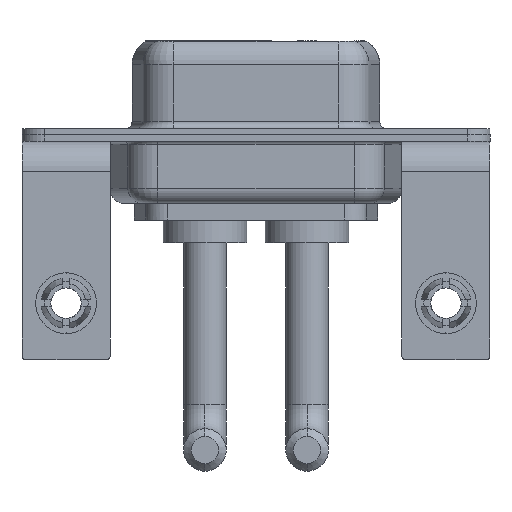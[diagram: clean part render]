
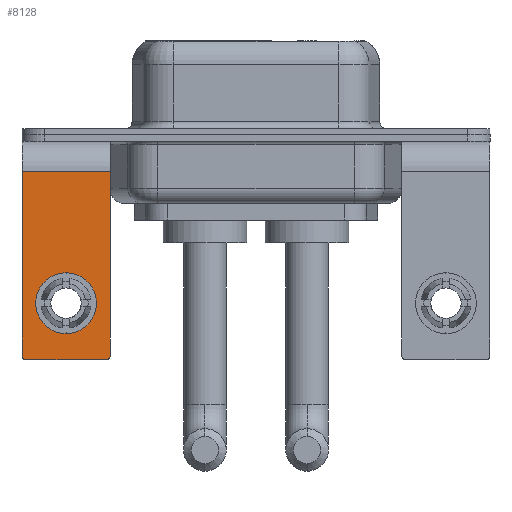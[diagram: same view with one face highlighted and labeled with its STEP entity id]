
A CAD part, front view. The second image highlights one B-rep face of the part: STEP entity #8128.
In plain terms, the highlighted planar face has unit normal (0, -1, 0).
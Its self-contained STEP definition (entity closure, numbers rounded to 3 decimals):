
#60 = VERTEX_POINT ( 'NONE', #4407 ) ;
#102 = EDGE_CURVE ( 'NONE', #496, #12610, #9292, .T. ) ;
#114 = ORIENTED_EDGE ( 'NONE', *, *, #12944, .T. ) ;
#496 = VERTEX_POINT ( 'NONE', #11418 ) ;
#649 = CIRCLE ( 'NONE', #12820, 2. ) ;
#994 = VERTEX_POINT ( 'NONE', #14543 ) ;
#1002 = DIRECTION ( 'NONE',  ( 0., 1., 0. ) ) ;
#1233 = ORIENTED_EDGE ( 'NONE', *, *, #102, .F. ) ;
#1258 = VERTEX_POINT ( 'NONE', #14523 ) ;
#1365 = DIRECTION ( 'NONE',  ( 0., 0., 1. ) ) ;
#1429 = EDGE_LOOP ( 'NONE', ( #15590, #114 ) ) ;
#1766 = ORIENTED_EDGE ( 'NONE', *, *, #7367, .T. ) ;
#1921 = CARTESIAN_POINT ( 'NONE',  ( 0., -6.25, -13.07 ) ) ;
#2092 = DIRECTION ( 'NONE',  ( -1., 0., 0. ) ) ;
#2646 = VECTOR ( 'NONE', #15547, 1000. ) ;
#2966 = CIRCLE ( 'NONE', #8007, 0.25 ) ;
#3191 = CIRCLE ( 'NONE', #12035, 0.25 ) ;
#3554 = EDGE_CURVE ( 'NONE', #1258, #60, #14537, .T. ) ;
#3587 = DIRECTION ( 'NONE',  ( 0., 0., -1. ) ) ;
#3794 = DIRECTION ( 'NONE',  ( 0., 0., 1. ) ) ;
#4407 = CARTESIAN_POINT ( 'NONE',  ( -2.9, -6.25, -2.4 ) ) ;
#4974 = CARTESIAN_POINT ( 'NONE',  ( 2.65, -6.25, -14.55 ) ) ;
#5122 = DIRECTION ( 'NONE',  ( 0., -1., 0. ) ) ;
#5253 = VECTOR ( 'NONE', #3587, 1000. ) ;
#6022 = EDGE_CURVE ( 'NONE', #496, #6179, #2966, .T. ) ;
#6058 = DIRECTION ( 'NONE',  ( 0., 0., 1. ) ) ;
#6179 = VERTEX_POINT ( 'NONE', #14928 ) ;
#6429 = DIRECTION ( 'NONE',  ( 0., 0., -1. ) ) ;
#6585 = CARTESIAN_POINT ( 'NONE',  ( -2.9, -6.25, -2.4 ) ) ;
#6658 = LINE ( 'NONE', #6585, #12731 ) ;
#7037 = PLANE ( 'NONE',  #14171 ) ;
#7367 = EDGE_CURVE ( 'NONE', #60, #14920, #6658, .T. ) ;
#7586 = CARTESIAN_POINT ( 'NONE',  ( -2.9, -6.25, -14.55 ) ) ;
#7698 = DIRECTION ( 'NONE',  ( 0., 0., 1. ) ) ;
#7740 = AXIS2_PLACEMENT_3D ( 'NONE', #13514, #11022, #6058 ) ;
#8007 = AXIS2_PLACEMENT_3D ( 'NONE', #4974, #5122, #3794 ) ;
#8128 = ADVANCED_FACE ( 'NONE', ( #9164, #14040 ), #7037, .F. ) ;
#8208 = CARTESIAN_POINT ( 'NONE',  ( 2.9, -6.25, -2.4 ) ) ;
#8475 = CARTESIAN_POINT ( 'NONE',  ( 2.9, -6.25, -2.4 ) ) ;
#8670 = CARTESIAN_POINT ( 'NONE',  ( -2.65, -6.25, -14.8 ) ) ;
#8759 = ORIENTED_EDGE ( 'NONE', *, *, #3554, .T. ) ;
#9117 = ORIENTED_EDGE ( 'NONE', *, *, #14228, .F. ) ;
#9119 = CARTESIAN_POINT ( 'NONE',  ( -2.65, -6.25, -14.55 ) ) ;
#9164 = FACE_BOUND ( 'NONE', #1429, .T. ) ;
#9292 = LINE ( 'NONE', #12957, #10881 ) ;
#9350 = CARTESIAN_POINT ( 'NONE',  ( 2.9, -6.25, -2.4 ) ) ;
#10291 = DIRECTION ( 'NONE',  ( 0., -1., 0. ) ) ;
#10802 = ORIENTED_EDGE ( 'NONE', *, *, #6022, .T. ) ;
#10862 = DIRECTION ( 'NONE',  ( 0., 1., 0. ) ) ;
#10881 = VECTOR ( 'NONE', #2092, 1000. ) ;
#11015 = CIRCLE ( 'NONE', #7740, 2. ) ;
#11022 = DIRECTION ( 'NONE',  ( 0., 1., 0. ) ) ;
#11418 = CARTESIAN_POINT ( 'NONE',  ( 2.65, -6.25, -14.8 ) ) ;
#11636 = DIRECTION ( 'NONE',  ( 0., 0., 1. ) ) ;
#11820 = LINE ( 'NONE', #9350, #5253 ) ;
#11872 = VERTEX_POINT ( 'NONE', #1921 ) ;
#12035 = AXIS2_PLACEMENT_3D ( 'NONE', #9119, #10291, #7698 ) ;
#12219 = CARTESIAN_POINT ( 'NONE',  ( 0., -6.25, -11.07 ) ) ;
#12610 = VERTEX_POINT ( 'NONE', #8670 ) ;
#12731 = VECTOR ( 'NONE', #6429, 1000. ) ;
#12820 = AXIS2_PLACEMENT_3D ( 'NONE', #12219, #10862, #1365 ) ;
#12944 = EDGE_CURVE ( 'NONE', #994, #11872, #649, .T. ) ;
#12957 = CARTESIAN_POINT ( 'NONE',  ( 2.9, -6.25, -14.8 ) ) ;
#12969 = EDGE_CURVE ( 'NONE', #11872, #994, #11015, .T. ) ;
#13086 = EDGE_LOOP ( 'NONE', ( #1766, #15259, #1233, #10802, #9117, #8759 ) ) ;
#13146 = EDGE_CURVE ( 'NONE', #14920, #12610, #3191, .T. ) ;
#13514 = CARTESIAN_POINT ( 'NONE',  ( 0., -6.25, -11.07 ) ) ;
#14040 = FACE_OUTER_BOUND ( 'NONE', #13086, .T. ) ;
#14171 = AXIS2_PLACEMENT_3D ( 'NONE', #8208, #1002, #11636 ) ;
#14228 = EDGE_CURVE ( 'NONE', #1258, #6179, #11820, .T. ) ;
#14523 = CARTESIAN_POINT ( 'NONE',  ( 2.9, -6.25, -2.4 ) ) ;
#14537 = LINE ( 'NONE', #8475, #2646 ) ;
#14543 = CARTESIAN_POINT ( 'NONE',  ( 0., -6.25, -9.07 ) ) ;
#14920 = VERTEX_POINT ( 'NONE', #7586 ) ;
#14928 = CARTESIAN_POINT ( 'NONE',  ( 2.9, -6.25, -14.55 ) ) ;
#15259 = ORIENTED_EDGE ( 'NONE', *, *, #13146, .T. ) ;
#15547 = DIRECTION ( 'NONE',  ( -1., 0., 0. ) ) ;
#15590 = ORIENTED_EDGE ( 'NONE', *, *, #12969, .T. ) ;
